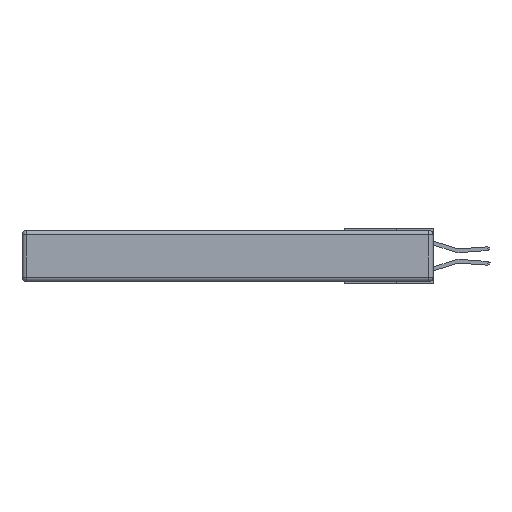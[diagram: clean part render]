
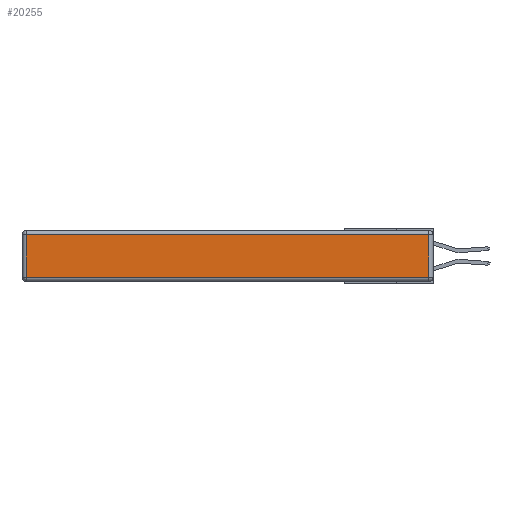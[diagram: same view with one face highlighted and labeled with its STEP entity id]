
A CAD part, left-side view. The second image highlights one B-rep face of the part: STEP entity #20255.
In plain terms, the highlighted planar face has unit normal (-1, 0, 0).
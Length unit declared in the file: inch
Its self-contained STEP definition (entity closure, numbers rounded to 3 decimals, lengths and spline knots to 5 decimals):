
#1693 = CARTESIAN_POINT ( 'NONE',  ( 0., 2.75, -0.03 ) ) ;
#1761 = EDGE_CURVE ( 'NONE', #17893, #16561, #2991, .T. ) ;
#2066 = LINE ( 'NONE', #1693, #9063 ) ;
#2585 = AXIS2_PLACEMENT_3D ( 'NONE', #8960, #3705, #3506 ) ;
#2598 = FACE_OUTER_BOUND ( 'NONE', #9574, .T. ) ;
#2991 = LINE ( 'NONE', #4924, #11933 ) ;
#3506 = DIRECTION ( 'NONE',  ( 0., 0., 1. ) ) ;
#3705 = DIRECTION ( 'NONE',  ( -1., 0., 0. ) ) ;
#4924 = CARTESIAN_POINT ( 'NONE',  ( 0., 0.03, -0.343 ) ) ;
#5392 = CARTESIAN_POINT ( 'NONE',  ( 0., 0.03, -0.03 ) ) ;
#6633 = ORIENTED_EDGE ( 'NONE', *, *, #24019, .T. ) ;
#6998 = CARTESIAN_POINT ( 'NONE',  ( 0., 0., -0.313 ) ) ;
#7763 = ORIENTED_EDGE ( 'NONE', *, *, #9906, .T. ) ;
#8114 = CARTESIAN_POINT ( 'NONE',  ( 0., 2.72, -0.313 ) ) ;
#8227 = CARTESIAN_POINT ( 'NONE',  ( 0., 0.03, -0.313 ) ) ;
#8504 = VERTEX_POINT ( 'NONE', #29164 ) ;
#8527 = PLANE ( 'NONE',  #2585 ) ;
#8960 = CARTESIAN_POINT ( 'NONE',  ( 0., 0., -0.343 ) ) ;
#9063 = VECTOR ( 'NONE', #31371, 39.37008 ) ;
#9574 = EDGE_LOOP ( 'NONE', ( #7763, #21793, #31956, #6633 ) ) ;
#9906 = EDGE_CURVE ( 'NONE', #22977, #17893, #15227, .T. ) ;
#11933 = VECTOR ( 'NONE', #22298, 39.37008 ) ;
#13827 = CARTESIAN_POINT ( 'NONE',  ( 0., 2.72, -0.343 ) ) ;
#15227 = LINE ( 'NONE', #6998, #17905 ) ;
#16561 = VERTEX_POINT ( 'NONE', #5392 ) ;
#17893 = VERTEX_POINT ( 'NONE', #8227 ) ;
#17905 = VECTOR ( 'NONE', #27216, 39.37008 ) ;
#20255 = ADVANCED_FACE ( 'NONE', ( #2598 ), #8527, .T. ) ;
#20723 = DIRECTION ( 'NONE',  ( 0., 0., -1. ) ) ;
#21793 = ORIENTED_EDGE ( 'NONE', *, *, #1761, .T. ) ;
#22298 = DIRECTION ( 'NONE',  ( 0., 0., 1. ) ) ;
#22797 = EDGE_CURVE ( 'NONE', #16561, #8504, #2066, .T. ) ;
#22977 = VERTEX_POINT ( 'NONE', #8114 ) ;
#24019 = EDGE_CURVE ( 'NONE', #8504, #22977, #29178, .T. ) ;
#27216 = DIRECTION ( 'NONE',  ( 0., -1., 0. ) ) ;
#28398 = VECTOR ( 'NONE', #20723, 39.37008 ) ;
#29164 = CARTESIAN_POINT ( 'NONE',  ( 0., 2.72, -0.03 ) ) ;
#29178 = LINE ( 'NONE', #13827, #28398 ) ;
#31371 = DIRECTION ( 'NONE',  ( 0., 1., 0. ) ) ;
#31956 = ORIENTED_EDGE ( 'NONE', *, *, #22797, .T. ) ;
